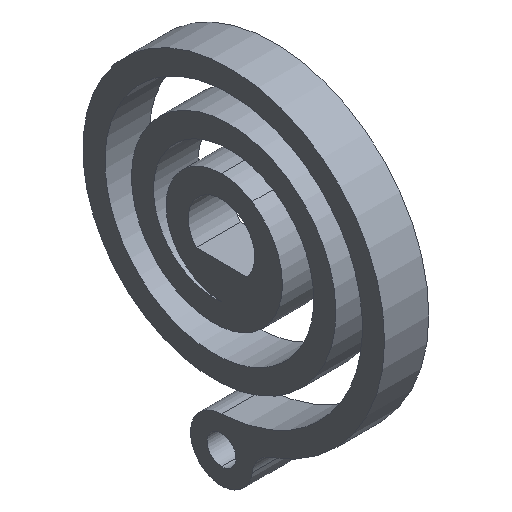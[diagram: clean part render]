
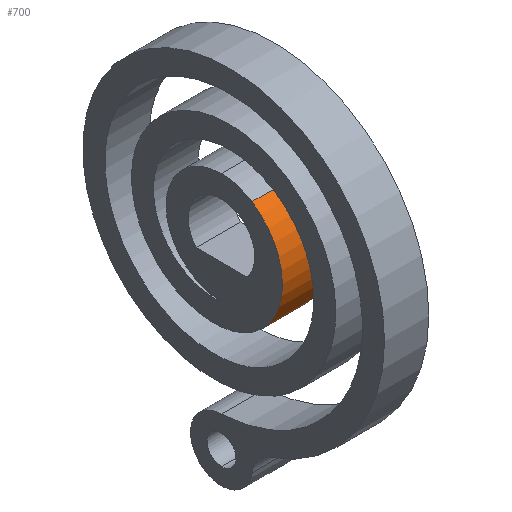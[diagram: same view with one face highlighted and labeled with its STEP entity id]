
A CAD part, isometric view. The second image highlights one B-rep face of the part: STEP entity #700.
In plain terms, the highlighted cylindrical face has radius 7.755 mm (diameter 15.51 mm), a partial arc.
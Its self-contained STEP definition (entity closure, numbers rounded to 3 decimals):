
#22 = AXIS2_PLACEMENT_3D ( 'NONE', #858, #861, #853 ) ;
#38 = CARTESIAN_POINT ( 'NONE',  ( 2.54, -3.489, 5.305 ) ) ;
#43 = CARTESIAN_POINT ( 'NONE',  ( 2.54, 0., -8.89 ) ) ;
#56 = CARTESIAN_POINT ( 'NONE',  ( -2.54, 0., -8.89 ) ) ;
#67 = EDGE_CURVE ( 'NONE', #848, #829, #439, .T. ) ;
#159 = EDGE_CURVE ( 'NONE', #618, #829, #374, .T. ) ;
#177 = EDGE_CURVE ( 'NONE', #857, #618, #414, .T. ) ;
#187 = DIRECTION ( 'NONE',  ( 0., 0., -1. ) ) ;
#269 = CYLINDRICAL_SURFACE ( 'NONE', #22, 7.755 ) ;
#271 = FACE_OUTER_BOUND ( 'NONE', #486, .T. ) ;
#286 = DIRECTION ( 'NONE',  ( 0., 0., -1. ) ) ;
#289 = DIRECTION ( 'NONE',  ( 1., 0., 0. ) ) ;
#292 = CARTESIAN_POINT ( 'NONE',  ( -2.54, 0.772, -1.174 ) ) ;
#296 = CARTESIAN_POINT ( 'NONE',  ( 2.54, -3.489, 5.305 ) ) ;
#315 = DIRECTION ( 'NONE',  ( -1., 0., 0. ) ) ;
#341 = DIRECTION ( 'NONE',  ( -1., 0., 0. ) ) ;
#342 = EDGE_CURVE ( 'NONE', #857, #848, #361, .T. ) ;
#353 = CARTESIAN_POINT ( 'NONE',  ( 2.54, 0.772, -1.174 ) ) ;
#361 = CIRCLE ( 'NONE', #925, 7.755 ) ;
#362 = VECTOR ( 'NONE', #315, 1000. ) ;
#374 = CIRCLE ( 'NONE', #481, 7.755 ) ;
#414 = LINE ( 'NONE', #296, #362 ) ;
#429 = VECTOR ( 'NONE', #341, 1000. ) ;
#439 = LINE ( 'NONE', #488, #429 ) ;
#466 = CARTESIAN_POINT ( 'NONE',  ( -2.54, -3.489, 5.305 ) ) ;
#481 = AXIS2_PLACEMENT_3D ( 'NONE', #292, #289, #286 ) ;
#486 = EDGE_LOOP ( 'NONE', ( #661, #667, #669, #670 ) ) ;
#488 = CARTESIAN_POINT ( 'NONE',  ( 2.54, 0., -8.89 ) ) ;
#618 = VERTEX_POINT ( 'NONE', #466 ) ;
#661 = ORIENTED_EDGE ( 'NONE', *, *, #159, .T. ) ;
#667 = ORIENTED_EDGE ( 'NONE', *, *, #67, .F. ) ;
#669 = ORIENTED_EDGE ( 'NONE', *, *, #342, .F. ) ;
#670 = ORIENTED_EDGE ( 'NONE', *, *, #177, .T. ) ;
#700 = ADVANCED_FACE ( 'NONE', ( #271 ), #269, .T. ) ;
#747 = DIRECTION ( 'NONE',  ( 1., 0., 0. ) ) ;
#829 = VERTEX_POINT ( 'NONE', #56 ) ;
#848 = VERTEX_POINT ( 'NONE', #43 ) ;
#853 = DIRECTION ( 'NONE',  ( 0., 0., 1. ) ) ;
#857 = VERTEX_POINT ( 'NONE', #38 ) ;
#858 = CARTESIAN_POINT ( 'NONE',  ( 2.54, 0.772, -1.174 ) ) ;
#861 = DIRECTION ( 'NONE',  ( -1., 0., 0. ) ) ;
#925 = AXIS2_PLACEMENT_3D ( 'NONE', #353, #747, #187 ) ;
